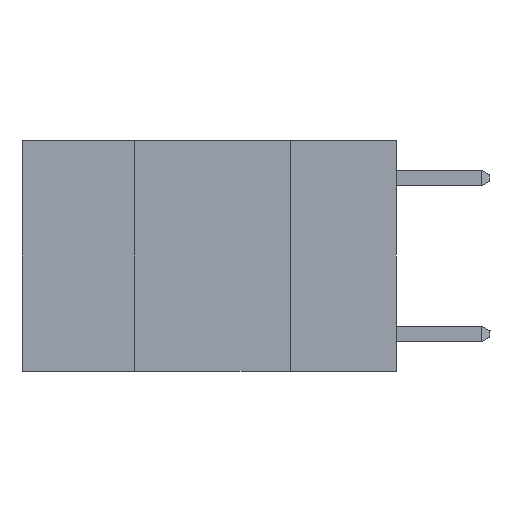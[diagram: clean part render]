
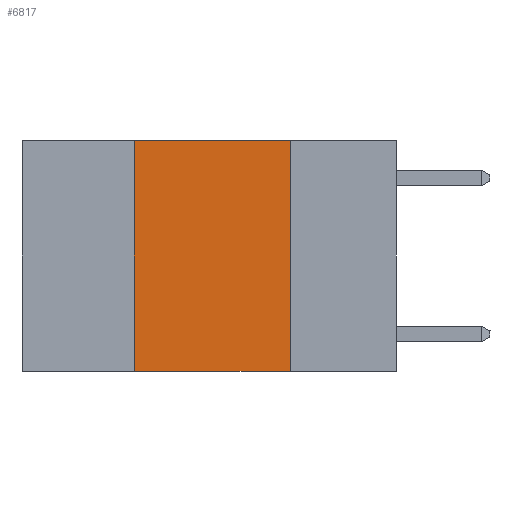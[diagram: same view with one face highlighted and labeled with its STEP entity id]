
A CAD part, left-side view. The second image highlights one B-rep face of the part: STEP entity #6817.
In plain terms, the highlighted planar face has unit normal (-1, 0, 0).
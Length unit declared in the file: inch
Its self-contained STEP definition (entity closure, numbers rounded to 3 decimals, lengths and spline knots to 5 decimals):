
#34 = ORIENTED_EDGE ( 'NONE', *, *, #8233, .T. ) ;
#638 = EDGE_CURVE ( 'NONE', #8052, #10322, #6681, .T. ) ;
#2587 = CARTESIAN_POINT ( 'NONE',  ( 0., 0.42, -0.37 ) ) ;
#2656 = EDGE_CURVE ( 'NONE', #11025, #6509, #4959, .T. ) ;
#3007 = DIRECTION ( 'NONE',  ( 1., 0., 0. ) ) ;
#3307 = DIRECTION ( 'NONE',  ( 0., 0., 1. ) ) ;
#3367 = CARTESIAN_POINT ( 'NONE',  ( 0., 0.42, 0. ) ) ;
#4076 = VECTOR ( 'NONE', #11445, 39.37008 ) ;
#4190 = EDGE_LOOP ( 'NONE', ( #4348, #10945, #10225, #34 ) ) ;
#4197 = EDGE_CURVE ( 'NONE', #6509, #8052, #8091, .T. ) ;
#4348 = ORIENTED_EDGE ( 'NONE', *, *, #638, .F. ) ;
#4467 = AXIS2_PLACEMENT_3D ( 'NONE', #8354, #3007, #9223 ) ;
#4959 = LINE ( 'NONE', #3367, #5278 ) ;
#5278 = VECTOR ( 'NONE', #3307, 39.37008 ) ;
#5283 = CARTESIAN_POINT ( 'NONE',  ( 0., 0.6, -0.37 ) ) ;
#5736 = DIRECTION ( 'NONE',  ( 0., 0., -1. ) ) ;
#6139 = CARTESIAN_POINT ( 'NONE',  ( 0., 0.17, 0. ) ) ;
#6509 = VERTEX_POINT ( 'NONE', #6910 ) ;
#6606 = FACE_OUTER_BOUND ( 'NONE', #4190, .T. ) ;
#6681 = LINE ( 'NONE', #6139, #6807 ) ;
#6807 = VECTOR ( 'NONE', #5736, 39.37008 ) ;
#6817 = ADVANCED_FACE ( 'NONE', ( #6606 ), #7443, .F. ) ;
#6910 = CARTESIAN_POINT ( 'NONE',  ( 0., 0.42, 0. ) ) ;
#7403 = DIRECTION ( 'NONE',  ( 0., -1., 0. ) ) ;
#7443 = PLANE ( 'NONE',  #4467 ) ;
#7963 = VECTOR ( 'NONE', #7403, 39.37008 ) ;
#8018 = CARTESIAN_POINT ( 'NONE',  ( 0., 0.6, 0. ) ) ;
#8052 = VERTEX_POINT ( 'NONE', #10280 ) ;
#8091 = LINE ( 'NONE', #8018, #7963 ) ;
#8233 = EDGE_CURVE ( 'NONE', #11025, #10322, #10875, .T. ) ;
#8354 = CARTESIAN_POINT ( 'NONE',  ( 0., 0.6, 0. ) ) ;
#9223 = DIRECTION ( 'NONE',  ( 0., 0., -1. ) ) ;
#9788 = CARTESIAN_POINT ( 'NONE',  ( 0., 0.17, -0.37 ) ) ;
#10225 = ORIENTED_EDGE ( 'NONE', *, *, #2656, .F. ) ;
#10280 = CARTESIAN_POINT ( 'NONE',  ( 0., 0.17, 0. ) ) ;
#10322 = VERTEX_POINT ( 'NONE', #9788 ) ;
#10875 = LINE ( 'NONE', #5283, #4076 ) ;
#10945 = ORIENTED_EDGE ( 'NONE', *, *, #4197, .F. ) ;
#11025 = VERTEX_POINT ( 'NONE', #2587 ) ;
#11445 = DIRECTION ( 'NONE',  ( 0., -1., 0. ) ) ;
